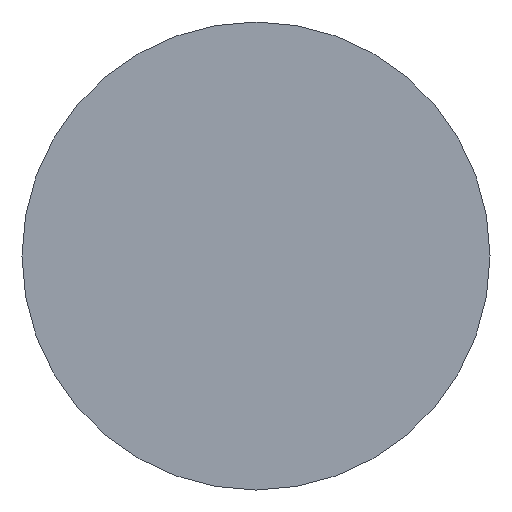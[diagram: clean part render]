
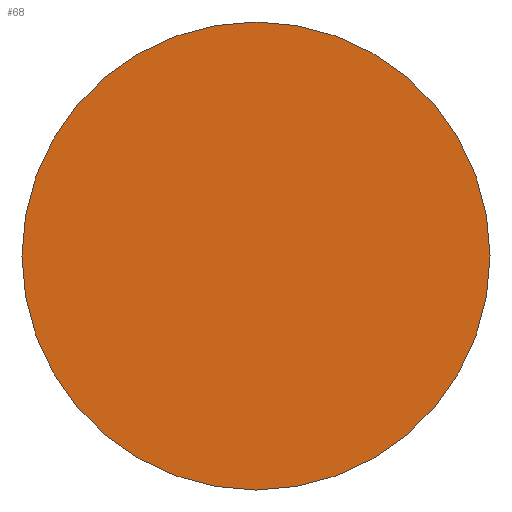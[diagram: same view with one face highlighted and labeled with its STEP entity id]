
A CAD part, left-side view. The second image highlights one B-rep face of the part: STEP entity #68.
In plain terms, the highlighted planar face has unit normal (-1, 0, 0).
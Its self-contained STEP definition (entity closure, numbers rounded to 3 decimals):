
#3 = CARTESIAN_POINT ( 'NONE',  ( 0., 0., 0. ) ) ;
#4 = DIRECTION ( 'NONE',  ( 1., 0., 0. ) ) ;
#6 = DIRECTION ( 'NONE',  ( 0., 0., -1. ) ) ;
#7 = DIRECTION ( 'NONE',  ( 1., 0., 0. ) ) ;
#9 = DIRECTION ( 'NONE',  ( 0., 0., -1. ) ) ;
#13 = CARTESIAN_POINT ( 'NONE',  ( 0., 0., 0. ) ) ;
#18 = CARTESIAN_POINT ( 'NONE',  ( 0., 0., -2. ) ) ;
#19 = CARTESIAN_POINT ( 'NONE',  ( 0., 0., 2. ) ) ;
#23 = DIRECTION ( 'NONE',  ( 1., 0., 0. ) ) ;
#24 = PLANE ( 'NONE',  #99 ) ;
#35 = CARTESIAN_POINT ( 'NONE',  ( 0., 0., 0. ) ) ;
#36 = DIRECTION ( 'NONE',  ( 0., 0., -1. ) ) ;
#68 = ADVANCED_FACE ( 'NONE', ( #165 ), #24, .F. ) ;
#69 = AXIS2_PLACEMENT_3D ( 'NONE', #3, #4, #9 ) ;
#75 = AXIS2_PLACEMENT_3D ( 'NONE', #13, #23, #36 ) ;
#95 = EDGE_CURVE ( 'NONE', #144, #155, #158, .T. ) ;
#98 = EDGE_CURVE ( 'NONE', #155, #144, #103, .T. ) ;
#99 = AXIS2_PLACEMENT_3D ( 'NONE', #35, #7, #6 ) ;
#103 = CIRCLE ( 'NONE', #69, 2. ) ;
#139 = ORIENTED_EDGE ( 'NONE', *, *, #95, .F. ) ;
#144 = VERTEX_POINT ( 'NONE', #19 ) ;
#145 = EDGE_LOOP ( 'NONE', ( #139, #151 ) ) ;
#151 = ORIENTED_EDGE ( 'NONE', *, *, #98, .F. ) ;
#155 = VERTEX_POINT ( 'NONE', #18 ) ;
#158 = CIRCLE ( 'NONE', #75, 2. ) ;
#165 = FACE_OUTER_BOUND ( 'NONE', #145, .T. ) ;
